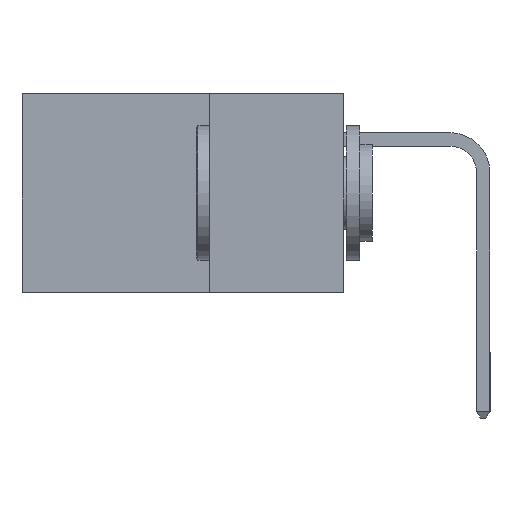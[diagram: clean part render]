
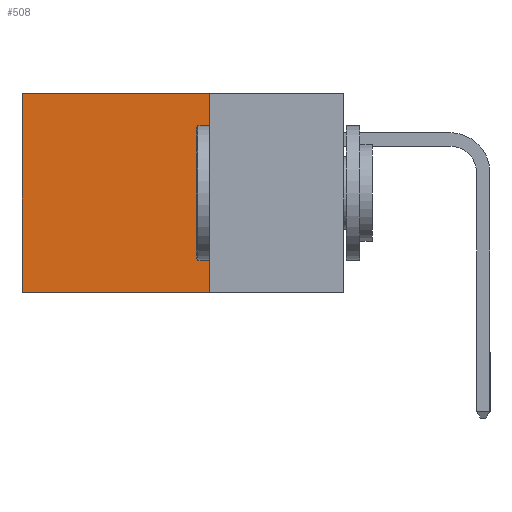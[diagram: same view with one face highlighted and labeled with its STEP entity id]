
A CAD part, left-side view. The second image highlights one B-rep face of the part: STEP entity #508.
In plain terms, the highlighted planar face has unit normal (-1, 0, 0).
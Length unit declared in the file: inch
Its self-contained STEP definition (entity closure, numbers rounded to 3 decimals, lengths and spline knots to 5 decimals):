
#393 = VERTEX_POINT ( 'NONE', #6859 ) ;
#479 = LINE ( 'NONE', #7932, #4054 ) ;
#505 = PLANE ( 'NONE',  #3145 ) ;
#508 = ADVANCED_FACE ( 'NONE', ( #2317 ), #505, .F. ) ;
#1323 = EDGE_CURVE ( 'NONE', #7913, #7791, #479, .T. ) ;
#1577 = DIRECTION ( 'NONE',  ( 0., 0., -1. ) ) ;
#1623 = VECTOR ( 'NONE', #2997, 39.37008 ) ;
#1812 = ORIENTED_EDGE ( 'NONE', *, *, #1323, .F. ) ;
#2317 = FACE_OUTER_BOUND ( 'NONE', #2491, .T. ) ;
#2491 = EDGE_LOOP ( 'NONE', ( #8707, #4977, #1812, #10189 ) ) ;
#2650 = EDGE_CURVE ( 'NONE', #7913, #393, #3563, .T. ) ;
#2843 = CARTESIAN_POINT ( 'NONE',  ( 0.2615, 0.25, 0. ) ) ;
#2997 = DIRECTION ( 'NONE',  ( 0., 1., 0. ) ) ;
#3145 = AXIS2_PLACEMENT_3D ( 'NONE', #8737, #6985, #8916 ) ;
#3255 = CARTESIAN_POINT ( 'NONE',  ( 0.2615, 0.25, -0.37 ) ) ;
#3563 = LINE ( 'NONE', #10031, #5220 ) ;
#3739 = LINE ( 'NONE', #3855, #1623 ) ;
#3855 = CARTESIAN_POINT ( 'NONE',  ( 0.2615, 0.25, -0.37 ) ) ;
#4054 = VECTOR ( 'NONE', #7020, 39.37008 ) ;
#4302 = CARTESIAN_POINT ( 'NONE',  ( 0.2615, 0.6, -0.37 ) ) ;
#4915 = EDGE_CURVE ( 'NONE', #393, #7407, #7562, .T. ) ;
#4977 = ORIENTED_EDGE ( 'NONE', *, *, #8833, .F. ) ;
#5220 = VECTOR ( 'NONE', #6256, 39.37008 ) ;
#6171 = CARTESIAN_POINT ( 'NONE',  ( 0.2615, 0.6, -0.37 ) ) ;
#6256 = DIRECTION ( 'NONE',  ( 0., 1., 0. ) ) ;
#6859 = CARTESIAN_POINT ( 'NONE',  ( 0.2615, 0.6, 0. ) ) ;
#6985 = DIRECTION ( 'NONE',  ( 1., 0., 0. ) ) ;
#7020 = DIRECTION ( 'NONE',  ( 0., 0., -1. ) ) ;
#7165 = VECTOR ( 'NONE', #1577, 39.37008 ) ;
#7407 = VERTEX_POINT ( 'NONE', #4302 ) ;
#7562 = LINE ( 'NONE', #6171, #7165 ) ;
#7791 = VERTEX_POINT ( 'NONE', #3255 ) ;
#7913 = VERTEX_POINT ( 'NONE', #2843 ) ;
#7932 = CARTESIAN_POINT ( 'NONE',  ( 0.2615, 0.25, -0.37 ) ) ;
#8707 = ORIENTED_EDGE ( 'NONE', *, *, #4915, .T. ) ;
#8737 = CARTESIAN_POINT ( 'NONE',  ( 0.2615, 0.25, -0.37 ) ) ;
#8833 = EDGE_CURVE ( 'NONE', #7791, #7407, #3739, .T. ) ;
#8916 = DIRECTION ( 'NONE',  ( 0., 0., -1. ) ) ;
#10031 = CARTESIAN_POINT ( 'NONE',  ( 0.2615, 0.25, 0. ) ) ;
#10189 = ORIENTED_EDGE ( 'NONE', *, *, #2650, .T. ) ;
